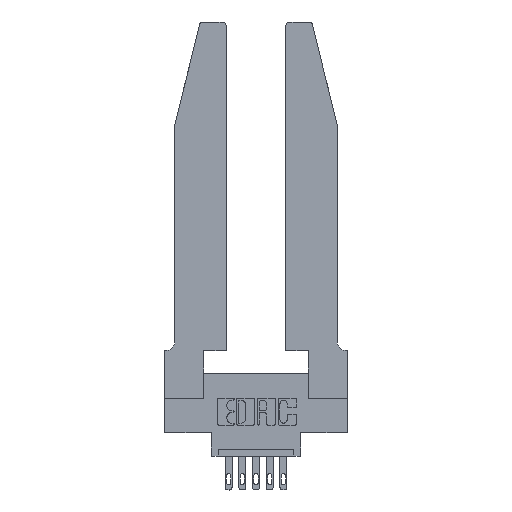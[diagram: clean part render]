
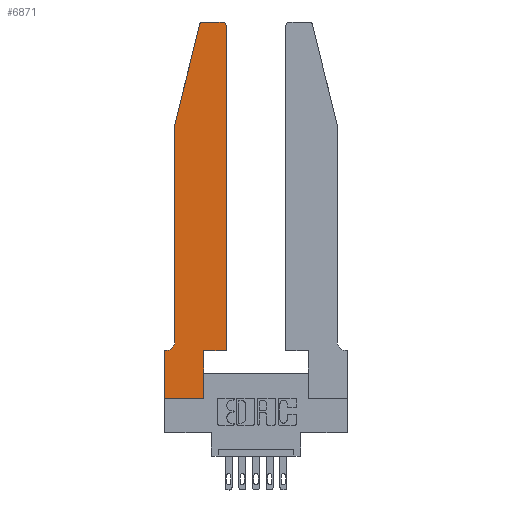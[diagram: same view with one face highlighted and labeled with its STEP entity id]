
A CAD part, top view. The second image highlights one B-rep face of the part: STEP entity #6871.
In plain terms, the highlighted planar face has unit normal (0, 0, 1).
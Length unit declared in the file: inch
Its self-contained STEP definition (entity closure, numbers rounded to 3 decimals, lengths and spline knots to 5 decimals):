
#80 = DIRECTION ( 'NONE',  ( 0., -1., 0. ) ) ;
#194 = CARTESIAN_POINT ( 'NONE',  ( 0.4505, 0.35, 0.37 ) ) ;
#354 = EDGE_CURVE ( 'NONE', #2192, #820, #11558, .T. ) ;
#432 = DIRECTION ( 'NONE',  ( 0., 0., 1. ) ) ;
#820 = VERTEX_POINT ( 'NONE', #10815 ) ;
#830 = VERTEX_POINT ( 'NONE', #4406 ) ;
#991 = EDGE_CURVE ( 'NONE', #7245, #11266, #12984, .T. ) ;
#1039 = AXIS2_PLACEMENT_3D ( 'NONE', #6723, #432, #3872 ) ;
#1048 = EDGE_CURVE ( 'NONE', #7464, #2192, #2168, .T. ) ;
#1567 = CARTESIAN_POINT ( 'NONE',  ( 0.4205, 2.75, 0.37 ) ) ;
#1660 = CARTESIAN_POINT ( 'NONE',  ( 0.2865, 0., 0.37 ) ) ;
#1790 = DIRECTION ( 'NONE',  ( 0., 0., -1. ) ) ;
#1963 = VERTEX_POINT ( 'NONE', #1660 ) ;
#2029 = CARTESIAN_POINT ( 'NONE',  ( 0.4505, 2.72, 0.37 ) ) ;
#2163 = CARTESIAN_POINT ( 'NONE',  ( 0.0055, 0.35, 0.37 ) ) ;
#2168 = LINE ( 'NONE', #6584, #10200 ) ;
#2172 = ORIENTED_EDGE ( 'NONE', *, *, #5479, .T. ) ;
#2192 = VERTEX_POINT ( 'NONE', #9678 ) ;
#2308 = EDGE_CURVE ( 'NONE', #7330, #1963, #8847, .T. ) ;
#2425 = DIRECTION ( 'NONE',  ( 1., 0., 0. ) ) ;
#2564 = EDGE_CURVE ( 'NONE', #13406, #3508, #6381, .T. ) ;
#2746 = ORIENTED_EDGE ( 'NONE', *, *, #9201, .T. ) ;
#2990 = DIRECTION ( 'NONE',  ( 0., 1., 0. ) ) ;
#2993 = ORIENTED_EDGE ( 'NONE', *, *, #1048, .T. ) ;
#3030 = ORIENTED_EDGE ( 'NONE', *, *, #2564, .T. ) ;
#3040 = AXIS2_PLACEMENT_3D ( 'NONE', #12751, #9692, #2425 ) ;
#3312 = VERTEX_POINT ( 'NONE', #10221 ) ;
#3508 = VERTEX_POINT ( 'NONE', #2029 ) ;
#3872 = DIRECTION ( 'NONE',  ( 1., 0., 0. ) ) ;
#3888 = DIRECTION ( 'NONE',  ( -1., 0., 0. ) ) ;
#4052 = CARTESIAN_POINT ( 'NONE',  ( 0.2865, 0.35, 0.37 ) ) ;
#4327 = ORIENTED_EDGE ( 'NONE', *, *, #10695, .T. ) ;
#4406 = CARTESIAN_POINT ( 'NONE',  ( 0.0755, 0.42, 0.37 ) ) ;
#4785 = CIRCLE ( 'NONE', #11616, 0.07 ) ;
#4830 = DIRECTION ( 'NONE',  ( 0., 0., 1. ) ) ;
#5092 = VERTEX_POINT ( 'NONE', #7612 ) ;
#5293 = CARTESIAN_POINT ( 'NONE',  ( 0.0755, 2., 0.37 ) ) ;
#5479 = EDGE_CURVE ( 'NONE', #1963, #3312, #11383, .T. ) ;
#5600 = VECTOR ( 'NONE', #12384, 39.37008 ) ;
#5718 = VECTOR ( 'NONE', #2990, 39.37008 ) ;
#5775 = DIRECTION ( 'NONE',  ( 1., 0., 0. ) ) ;
#6042 = VECTOR ( 'NONE', #11741, 39.37008 ) ;
#6110 = VECTOR ( 'NONE', #80, 39.37008 ) ;
#6113 = FACE_OUTER_BOUND ( 'NONE', #7062, .T. ) ;
#6126 = VECTOR ( 'NONE', #9632, 39.37008 ) ;
#6132 = ORIENTED_EDGE ( 'NONE', *, *, #2308, .T. ) ;
#6381 = LINE ( 'NONE', #9316, #5718 ) ;
#6460 = ORIENTED_EDGE ( 'NONE', *, *, #10245, .T. ) ;
#6584 = CARTESIAN_POINT ( 'NONE',  ( 0.2605, 2.75, 0.37 ) ) ;
#6589 = EDGE_CURVE ( 'NONE', #820, #5092, #9262, .T. ) ;
#6618 = LINE ( 'NONE', #5293, #6110 ) ;
#6723 = CARTESIAN_POINT ( 'NONE',  ( 0.4205, 2.72, 0.37 ) ) ;
#6871 = ADVANCED_FACE ( 'NONE', ( #6113 ), #11130, .T. ) ;
#6914 = VECTOR ( 'NONE', #8219, 39.37008 ) ;
#6993 = CARTESIAN_POINT ( 'NONE',  ( 0.0055, 0.42, 0.37 ) ) ;
#7001 = CARTESIAN_POINT ( 'NONE',  ( 0., 0.35, 0.37 ) ) ;
#7062 = EDGE_LOOP ( 'NONE', ( #2993, #8194, #12997, #12954, #2746, #10172, #6460, #6132, #2172, #8082, #3030, #4327 ) ) ;
#7174 = CARTESIAN_POINT ( 'NONE',  ( 0., 0., 0.37 ) ) ;
#7239 = CARTESIAN_POINT ( 'NONE',  ( 0.4505, 0.35, 0.37 ) ) ;
#7245 = VERTEX_POINT ( 'NONE', #2163 ) ;
#7264 = DIRECTION ( 'NONE',  ( 0., 1., 0. ) ) ;
#7330 = VERTEX_POINT ( 'NONE', #12823 ) ;
#7464 = VERTEX_POINT ( 'NONE', #1567 ) ;
#7612 = CARTESIAN_POINT ( 'NONE',  ( 0.0755, 2., 0.37 ) ) ;
#8082 = ORIENTED_EDGE ( 'NONE', *, *, #10569, .T. ) ;
#8105 = VECTOR ( 'NONE', #7264, 39.37008 ) ;
#8194 = ORIENTED_EDGE ( 'NONE', *, *, #354, .T. ) ;
#8219 = DIRECTION ( 'NONE',  ( 0., -1., 0. ) ) ;
#8487 = CARTESIAN_POINT ( 'NONE',  ( 0., 0., 0.37 ) ) ;
#8592 = CARTESIAN_POINT ( 'NONE',  ( 0.0755, 2., 0.37 ) ) ;
#8847 = LINE ( 'NONE', #8487, #6042 ) ;
#8969 = EDGE_CURVE ( 'NONE', #5092, #830, #6618, .T. ) ;
#9201 = EDGE_CURVE ( 'NONE', #830, #7245, #4785, .T. ) ;
#9210 = CARTESIAN_POINT ( 'NONE',  ( 0.0755, 0.35, 0.37 ) ) ;
#9221 = LINE ( 'NONE', #7174, #6914 ) ;
#9262 = LINE ( 'NONE', #8592, #6126 ) ;
#9316 = CARTESIAN_POINT ( 'NONE',  ( 0.4505, 0.35, 0.37 ) ) ;
#9330 = AXIS2_PLACEMENT_3D ( 'NONE', #7001, #4830, #5775 ) ;
#9525 = VECTOR ( 'NONE', #10685, 39.37008 ) ;
#9558 = DIRECTION ( 'NONE',  ( -1., 0., 0. ) ) ;
#9632 = DIRECTION ( 'NONE',  ( -0.239, -0.971, 0. ) ) ;
#9678 = CARTESIAN_POINT ( 'NONE',  ( 0.284, 2.75, 0.37 ) ) ;
#9692 = DIRECTION ( 'NONE',  ( 0., 0., 1. ) ) ;
#10172 = ORIENTED_EDGE ( 'NONE', *, *, #991, .T. ) ;
#10200 = VECTOR ( 'NONE', #9558, 39.37008 ) ;
#10221 = CARTESIAN_POINT ( 'NONE',  ( 0.2865, 0.35, 0.37 ) ) ;
#10245 = EDGE_CURVE ( 'NONE', #11266, #7330, #9221, .T. ) ;
#10569 = EDGE_CURVE ( 'NONE', #3312, #13406, #12291, .T. ) ;
#10650 = CIRCLE ( 'NONE', #1039, 0.03 ) ;
#10685 = DIRECTION ( 'NONE',  ( 1., 0., 0. ) ) ;
#10695 = EDGE_CURVE ( 'NONE', #3508, #7464, #10650, .T. ) ;
#10815 = CARTESIAN_POINT ( 'NONE',  ( 0.25487, 2.72718, 0.37 ) ) ;
#11130 = PLANE ( 'NONE',  #9330 ) ;
#11266 = VERTEX_POINT ( 'NONE', #12311 ) ;
#11383 = LINE ( 'NONE', #4052, #8105 ) ;
#11558 = CIRCLE ( 'NONE', #3040, 0.03 ) ;
#11616 = AXIS2_PLACEMENT_3D ( 'NONE', #6993, #1790, #3888 ) ;
#11741 = DIRECTION ( 'NONE',  ( 1., 0., 0. ) ) ;
#12291 = LINE ( 'NONE', #194, #9525 ) ;
#12311 = CARTESIAN_POINT ( 'NONE',  ( 0., 0.35, 0.37 ) ) ;
#12384 = DIRECTION ( 'NONE',  ( -1., 0., 0. ) ) ;
#12751 = CARTESIAN_POINT ( 'NONE',  ( 0.284, 2.72, 0.37 ) ) ;
#12823 = CARTESIAN_POINT ( 'NONE',  ( 0., 0., 0.37 ) ) ;
#12954 = ORIENTED_EDGE ( 'NONE', *, *, #8969, .T. ) ;
#12984 = LINE ( 'NONE', #9210, #5600 ) ;
#12997 = ORIENTED_EDGE ( 'NONE', *, *, #6589, .T. ) ;
#13406 = VERTEX_POINT ( 'NONE', #7239 ) ;
